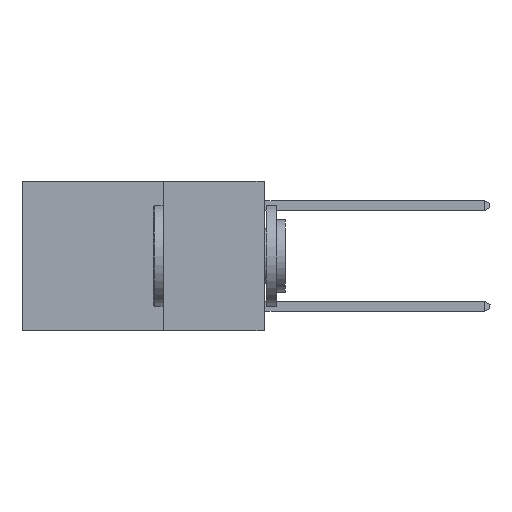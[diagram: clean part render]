
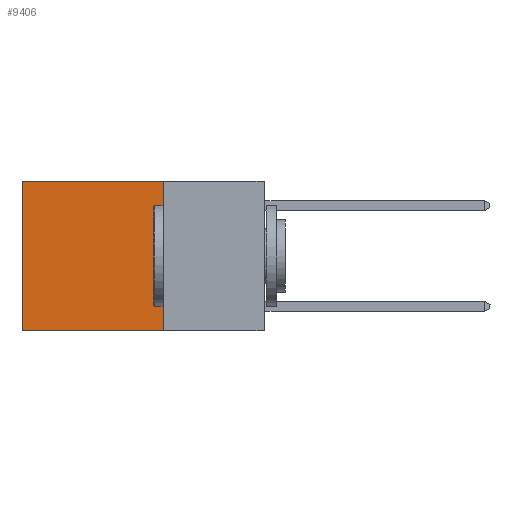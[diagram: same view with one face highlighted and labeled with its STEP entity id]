
A CAD part, left-side view. The second image highlights one B-rep face of the part: STEP entity #9406.
In plain terms, the highlighted planar face has unit normal (-1, 0, 0).
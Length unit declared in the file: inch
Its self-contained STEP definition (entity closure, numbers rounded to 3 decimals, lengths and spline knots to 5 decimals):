
#220 = LINE ( 'NONE', #5833, #6694 ) ;
#522 = VERTEX_POINT ( 'NONE', #10322 ) ;
#748 = PLANE ( 'NONE',  #3260 ) ;
#879 = DIRECTION ( 'NONE',  ( 0., 0., -1. ) ) ;
#890 = EDGE_CURVE ( 'NONE', #2722, #522, #220, .T. ) ;
#1088 = VECTOR ( 'NONE', #8947, 39.37008 ) ;
#1357 = CARTESIAN_POINT ( 'NONE',  ( 0.2625, 0.6, 0. ) ) ;
#1508 = VECTOR ( 'NONE', #4330, 39.37008 ) ;
#1790 = CARTESIAN_POINT ( 'NONE',  ( 0.2625, 0.25, -0.37 ) ) ;
#2180 = EDGE_CURVE ( 'NONE', #522, #6326, #3819, .T. ) ;
#2722 = VERTEX_POINT ( 'NONE', #3126 ) ;
#2974 = CARTESIAN_POINT ( 'NONE',  ( 0.2625, 0.6, -0.37 ) ) ;
#3126 = CARTESIAN_POINT ( 'NONE',  ( 0.2625, 0.25, 0. ) ) ;
#3260 = AXIS2_PLACEMENT_3D ( 'NONE', #8389, #10024, #5006 ) ;
#3420 = ORIENTED_EDGE ( 'NONE', *, *, #6747, .F. ) ;
#3748 = LINE ( 'NONE', #1790, #1508 ) ;
#3819 = LINE ( 'NONE', #1357, #8372 ) ;
#3838 = CARTESIAN_POINT ( 'NONE',  ( 0.2625, 0.25, 0. ) ) ;
#3869 = EDGE_LOOP ( 'NONE', ( #8853, #3420, #4176, #3955 ) ) ;
#3955 = ORIENTED_EDGE ( 'NONE', *, *, #890, .T. ) ;
#4176 = ORIENTED_EDGE ( 'NONE', *, *, #10479, .F. ) ;
#4330 = DIRECTION ( 'NONE',  ( 0., 1., 0. ) ) ;
#5006 = DIRECTION ( 'NONE',  ( 0., 0., -1. ) ) ;
#5356 = VERTEX_POINT ( 'NONE', #10119 ) ;
#5618 = LINE ( 'NONE', #3838, #1088 ) ;
#5833 = CARTESIAN_POINT ( 'NONE',  ( 0.2625, 0.25, 0. ) ) ;
#6326 = VERTEX_POINT ( 'NONE', #2974 ) ;
#6694 = VECTOR ( 'NONE', #8227, 39.37008 ) ;
#6747 = EDGE_CURVE ( 'NONE', #5356, #6326, #3748, .T. ) ;
#8227 = DIRECTION ( 'NONE',  ( 0., 1., 0. ) ) ;
#8372 = VECTOR ( 'NONE', #879, 39.37008 ) ;
#8389 = CARTESIAN_POINT ( 'NONE',  ( 0.2625, 0.25, 0. ) ) ;
#8693 = FACE_OUTER_BOUND ( 'NONE', #3869, .T. ) ;
#8853 = ORIENTED_EDGE ( 'NONE', *, *, #2180, .T. ) ;
#8947 = DIRECTION ( 'NONE',  ( 0., 0., -1. ) ) ;
#9406 = ADVANCED_FACE ( 'NONE', ( #8693 ), #748, .F. ) ;
#10024 = DIRECTION ( 'NONE',  ( 1., 0., 0. ) ) ;
#10119 = CARTESIAN_POINT ( 'NONE',  ( 0.2625, 0.25, -0.37 ) ) ;
#10322 = CARTESIAN_POINT ( 'NONE',  ( 0.2625, 0.6, 0. ) ) ;
#10479 = EDGE_CURVE ( 'NONE', #2722, #5356, #5618, .T. ) ;
